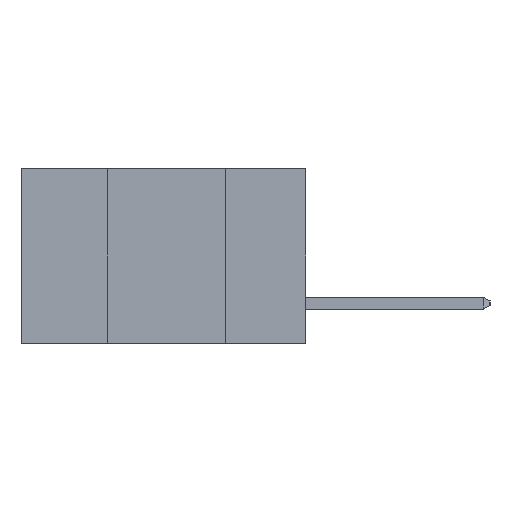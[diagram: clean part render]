
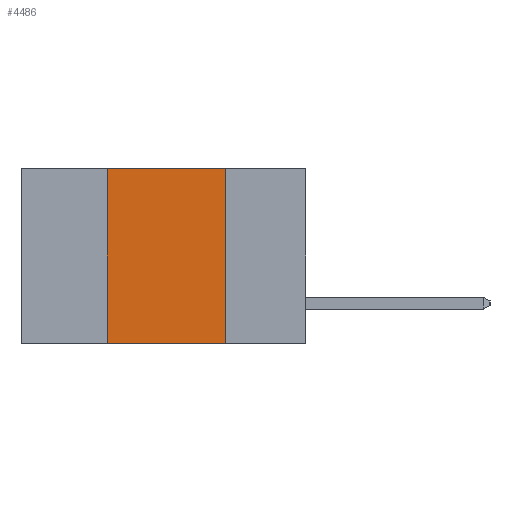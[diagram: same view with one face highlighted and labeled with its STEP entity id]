
A CAD part, left-side view. The second image highlights one B-rep face of the part: STEP entity #4486.
In plain terms, the highlighted planar face has unit normal (-1, 0, 0).
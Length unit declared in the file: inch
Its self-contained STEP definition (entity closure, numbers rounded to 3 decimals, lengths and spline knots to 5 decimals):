
#280 = DIRECTION ( 'NONE',  ( 0., -1., 0. ) ) ;
#602 = AXIS2_PLACEMENT_3D ( 'NONE', #7819, #9862, #3648 ) ;
#1456 = ORIENTED_EDGE ( 'NONE', *, *, #10709, .F. ) ;
#1506 = CARTESIAN_POINT ( 'NONE',  ( 0., 0.17, 0. ) ) ;
#1584 = VECTOR ( 'NONE', #10534, 39.37008 ) ;
#1819 = ORIENTED_EDGE ( 'NONE', *, *, #2595, .F. ) ;
#2595 = EDGE_CURVE ( 'NONE', #2944, #11549, #8066, .T. ) ;
#2910 = VECTOR ( 'NONE', #280, 39.37008 ) ;
#2944 = VERTEX_POINT ( 'NONE', #6494 ) ;
#3648 = DIRECTION ( 'NONE',  ( 0., 0., -1. ) ) ;
#3812 = LINE ( 'NONE', #12084, #11637 ) ;
#4486 = ADVANCED_FACE ( 'NONE', ( #6459 ), #8846, .F. ) ;
#4543 = EDGE_CURVE ( 'NONE', #9679, #11959, #11142, .T. ) ;
#5000 = DIRECTION ( 'NONE',  ( 0., 0., 1. ) ) ;
#6459 = FACE_OUTER_BOUND ( 'NONE', #12504, .T. ) ;
#6494 = CARTESIAN_POINT ( 'NONE',  ( 0., 0.42, 0. ) ) ;
#7819 = CARTESIAN_POINT ( 'NONE',  ( 0., 0.6, 0. ) ) ;
#8066 = LINE ( 'NONE', #9993, #10446 ) ;
#8130 = ORIENTED_EDGE ( 'NONE', *, *, #4543, .T. ) ;
#8846 = PLANE ( 'NONE',  #602 ) ;
#9679 = VERTEX_POINT ( 'NONE', #13214 ) ;
#9812 = EDGE_CURVE ( 'NONE', #11549, #11959, #13148, .T. ) ;
#9862 = DIRECTION ( 'NONE',  ( 1., 0., 0. ) ) ;
#9883 = ORIENTED_EDGE ( 'NONE', *, *, #9812, .F. ) ;
#9903 = CARTESIAN_POINT ( 'NONE',  ( 0., 0.6, -0.37 ) ) ;
#9948 = DIRECTION ( 'NONE',  ( 0., -1., 0. ) ) ;
#9993 = CARTESIAN_POINT ( 'NONE',  ( 0., 0.6, 0. ) ) ;
#10446 = VECTOR ( 'NONE', #9948, 39.37008 ) ;
#10534 = DIRECTION ( 'NONE',  ( 0., 0., -1. ) ) ;
#10709 = EDGE_CURVE ( 'NONE', #9679, #2944, #3812, .T. ) ;
#11142 = LINE ( 'NONE', #9903, #2910 ) ;
#11549 = VERTEX_POINT ( 'NONE', #1506 ) ;
#11637 = VECTOR ( 'NONE', #5000, 39.37008 ) ;
#11959 = VERTEX_POINT ( 'NONE', #13487 ) ;
#12084 = CARTESIAN_POINT ( 'NONE',  ( 0., 0.42, 0. ) ) ;
#12468 = CARTESIAN_POINT ( 'NONE',  ( 0., 0.17, 0. ) ) ;
#12504 = EDGE_LOOP ( 'NONE', ( #9883, #1819, #1456, #8130 ) ) ;
#13148 = LINE ( 'NONE', #12468, #1584 ) ;
#13214 = CARTESIAN_POINT ( 'NONE',  ( 0., 0.42, -0.37 ) ) ;
#13487 = CARTESIAN_POINT ( 'NONE',  ( 0., 0.17, -0.37 ) ) ;
